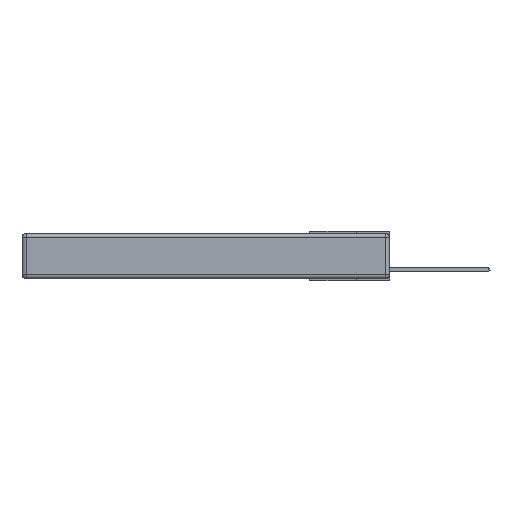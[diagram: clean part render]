
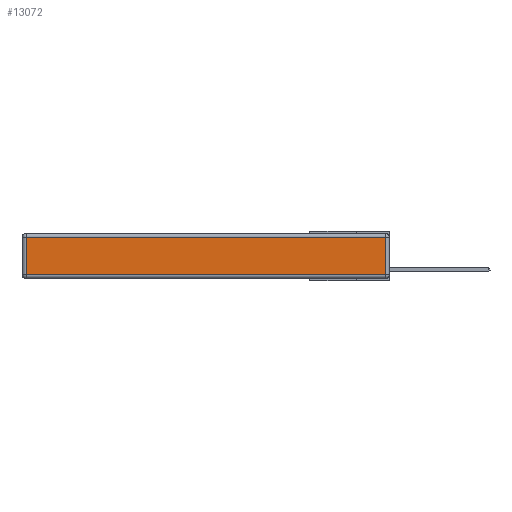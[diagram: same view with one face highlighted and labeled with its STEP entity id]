
A CAD part, left-side view. The second image highlights one B-rep face of the part: STEP entity #13072.
In plain terms, the highlighted planar face has unit normal (-1, 0, 0).
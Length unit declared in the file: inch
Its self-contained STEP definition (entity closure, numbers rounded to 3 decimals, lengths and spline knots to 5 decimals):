
#43 = ORIENTED_EDGE ( 'NONE', *, *, #17626, .T. ) ;
#911 = LINE ( 'NONE', #4507, #4832 ) ;
#1501 = ORIENTED_EDGE ( 'NONE', *, *, #10899, .T. ) ;
#1557 = PLANE ( 'NONE',  #17942 ) ;
#1774 = EDGE_CURVE ( 'NONE', #7306, #6328, #12156, .T. ) ;
#2167 = DIRECTION ( 'NONE',  ( 0., 0., 1. ) ) ;
#3555 = VERTEX_POINT ( 'NONE', #8175 ) ;
#3592 = VERTEX_POINT ( 'NONE', #7656 ) ;
#4507 = CARTESIAN_POINT ( 'NONE',  ( 0., 2.72, -0.343 ) ) ;
#4832 = VECTOR ( 'NONE', #13278, 39.37008 ) ;
#4839 = ORIENTED_EDGE ( 'NONE', *, *, #8323, .T. ) ;
#6328 = VERTEX_POINT ( 'NONE', #9525 ) ;
#7306 = VERTEX_POINT ( 'NONE', #10141 ) ;
#7411 = DIRECTION ( 'NONE',  ( -1., 0., 0. ) ) ;
#7656 = CARTESIAN_POINT ( 'NONE',  ( 0., 2.72, -0.03 ) ) ;
#7681 = CARTESIAN_POINT ( 'NONE',  ( 0., 2.75, -0.03 ) ) ;
#7735 = CARTESIAN_POINT ( 'NONE',  ( 0., 0., -0.313 ) ) ;
#8175 = CARTESIAN_POINT ( 'NONE',  ( 0., 0.03, -0.03 ) ) ;
#8212 = VECTOR ( 'NONE', #18115, 39.37008 ) ;
#8323 = EDGE_CURVE ( 'NONE', #6328, #3555, #18632, .T. ) ;
#8462 = FACE_OUTER_BOUND ( 'NONE', #14482, .T. ) ;
#9525 = CARTESIAN_POINT ( 'NONE',  ( 0., 0.03, -0.313 ) ) ;
#10141 = CARTESIAN_POINT ( 'NONE',  ( 0., 2.72, -0.313 ) ) ;
#10716 = VECTOR ( 'NONE', #17996, 39.37008 ) ;
#10899 = EDGE_CURVE ( 'NONE', #3555, #3592, #17394, .T. ) ;
#11886 = DIRECTION ( 'NONE',  ( 0., 0., 1. ) ) ;
#12156 = LINE ( 'NONE', #7735, #8212 ) ;
#13072 = ADVANCED_FACE ( 'NONE', ( #8462 ), #1557, .T. ) ;
#13278 = DIRECTION ( 'NONE',  ( 0., 0., -1. ) ) ;
#14252 = VECTOR ( 'NONE', #2167, 39.37008 ) ;
#14482 = EDGE_LOOP ( 'NONE', ( #14890, #4839, #1501, #43 ) ) ;
#14890 = ORIENTED_EDGE ( 'NONE', *, *, #1774, .T. ) ;
#14904 = CARTESIAN_POINT ( 'NONE',  ( 0., 0., -0.343 ) ) ;
#16347 = CARTESIAN_POINT ( 'NONE',  ( 0., 0.03, -0.343 ) ) ;
#17394 = LINE ( 'NONE', #7681, #10716 ) ;
#17626 = EDGE_CURVE ( 'NONE', #3592, #7306, #911, .T. ) ;
#17942 = AXIS2_PLACEMENT_3D ( 'NONE', #14904, #7411, #11886 ) ;
#17996 = DIRECTION ( 'NONE',  ( 0., 1., 0. ) ) ;
#18115 = DIRECTION ( 'NONE',  ( 0., -1., 0. ) ) ;
#18632 = LINE ( 'NONE', #16347, #14252 ) ;
